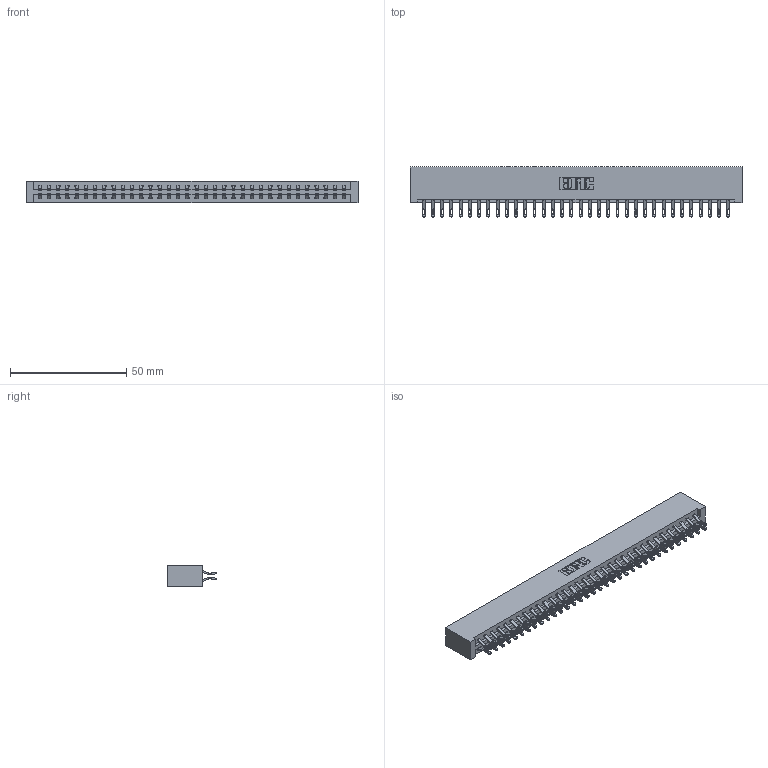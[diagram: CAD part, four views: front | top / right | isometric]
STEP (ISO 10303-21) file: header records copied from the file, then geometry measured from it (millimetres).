
FILE_DESCRIPTION (( 'STEP AP203' ), '1' );
FILE_NAME ('337-068-555-201.STEP', '2018-08-11T10:28:54', ( '' ), ( '' ), 'SwSTEP 2.0', 'SolidWorks 2016', '' );
FILE_SCHEMA (( 'CONFIG_CONTROL_DESIGN' ));
Length unit declared in the file: inch
Products named in the file (3): 337 Part_No Mounting Lugs; 345-292-001_555 Tail; 337-068-555-201
Assembly tree (69 placements, depth 2):
  337-068-555-201
    337 Part_No Mounting Lugs
    345-292-001_555 Tail  x68
Bounding box: 142.6 x 21.47 x 9.4 mm (x, y, z)
Volume: 15879.3 mm3; surface area: 18673.3 mm2
Topology: 69 solids, 69 shells, 4186 faces, 13139 edges, 8758 vertices
Faces by surface type: plane 2514, cylinder 1672
Entity records: 27445 total; most frequent: CARTESIAN_POINT 4664, ORIENTED_EDGE 4570, DIRECTION 3945, EDGE_CURVE 2285, LINE 2145, VECTOR 2145, VERTEX_POINT 1522, AXIS2_PLACEMENT_3D 900
